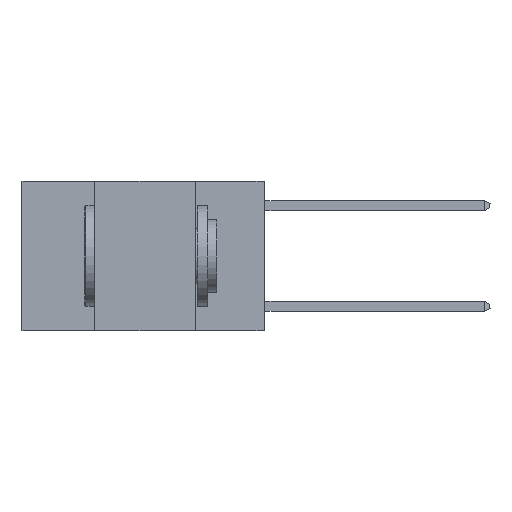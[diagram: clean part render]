
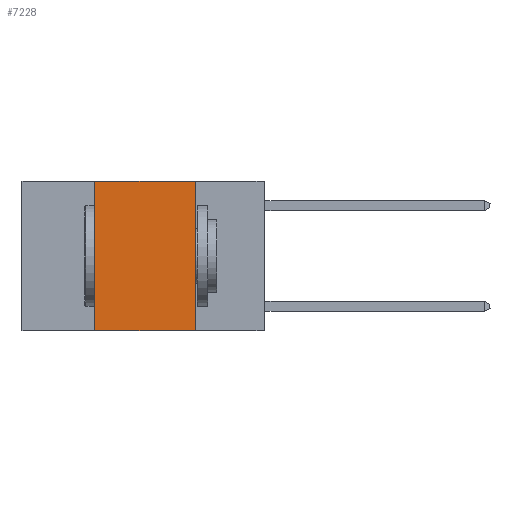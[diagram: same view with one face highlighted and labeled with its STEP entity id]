
A CAD part, left-side view. The second image highlights one B-rep face of the part: STEP entity #7228.
In plain terms, the highlighted planar face has unit normal (-1, 0, 0).
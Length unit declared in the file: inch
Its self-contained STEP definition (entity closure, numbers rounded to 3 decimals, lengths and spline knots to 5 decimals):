
#251 = VECTOR ( 'NONE', #2437, 39.37008 ) ;
#270 = EDGE_CURVE ( 'NONE', #9111, #2203, #6574, .T. ) ;
#506 = EDGE_LOOP ( 'NONE', ( #3416, #1735, #6594, #8773 ) ) ;
#583 = VECTOR ( 'NONE', #8448, 39.37008 ) ;
#635 = FACE_OUTER_BOUND ( 'NONE', #506, .T. ) ;
#727 = CARTESIAN_POINT ( 'NONE',  ( 0., 0.17, 0. ) ) ;
#1605 = CARTESIAN_POINT ( 'NONE',  ( 0., 0.17, -0.37 ) ) ;
#1732 = CARTESIAN_POINT ( 'NONE',  ( 0., 0.42, -0.37 ) ) ;
#1735 = ORIENTED_EDGE ( 'NONE', *, *, #2881, .F. ) ;
#2203 = VERTEX_POINT ( 'NONE', #5775 ) ;
#2244 = DIRECTION ( 'NONE',  ( 0., 0., 1. ) ) ;
#2437 = DIRECTION ( 'NONE',  ( 0., 0., -1. ) ) ;
#2881 = EDGE_CURVE ( 'NONE', #2203, #7790, #3238, .T. ) ;
#3238 = LINE ( 'NONE', #8332, #583 ) ;
#3416 = ORIENTED_EDGE ( 'NONE', *, *, #10229, .F. ) ;
#3858 = DIRECTION ( 'NONE',  ( 0., -1., 0. ) ) ;
#3930 = DIRECTION ( 'NONE',  ( 1., 0., 0. ) ) ;
#3982 = VECTOR ( 'NONE', #2244, 39.37008 ) ;
#4307 = VECTOR ( 'NONE', #3858, 39.37008 ) ;
#4714 = DIRECTION ( 'NONE',  ( 0., 0., -1. ) ) ;
#4939 = PLANE ( 'NONE',  #5691 ) ;
#5344 = LINE ( 'NONE', #9527, #251 ) ;
#5599 = CARTESIAN_POINT ( 'NONE',  ( 0., 0.6, -0.37 ) ) ;
#5691 = AXIS2_PLACEMENT_3D ( 'NONE', #7385, #3930, #4714 ) ;
#5775 = CARTESIAN_POINT ( 'NONE',  ( 0., 0.42, 0. ) ) ;
#6574 = LINE ( 'NONE', #10867, #3982 ) ;
#6594 = ORIENTED_EDGE ( 'NONE', *, *, #270, .F. ) ;
#7228 = ADVANCED_FACE ( 'NONE', ( #635 ), #4939, .F. ) ;
#7385 = CARTESIAN_POINT ( 'NONE',  ( 0., 0.6, 0. ) ) ;
#7790 = VERTEX_POINT ( 'NONE', #727 ) ;
#8332 = CARTESIAN_POINT ( 'NONE',  ( 0., 0.6, 0. ) ) ;
#8448 = DIRECTION ( 'NONE',  ( 0., -1., 0. ) ) ;
#8773 = ORIENTED_EDGE ( 'NONE', *, *, #10844, .T. ) ;
#8787 = LINE ( 'NONE', #5599, #4307 ) ;
#9111 = VERTEX_POINT ( 'NONE', #1732 ) ;
#9527 = CARTESIAN_POINT ( 'NONE',  ( 0., 0.17, 0. ) ) ;
#9935 = VERTEX_POINT ( 'NONE', #1605 ) ;
#10229 = EDGE_CURVE ( 'NONE', #7790, #9935, #5344, .T. ) ;
#10844 = EDGE_CURVE ( 'NONE', #9111, #9935, #8787, .T. ) ;
#10867 = CARTESIAN_POINT ( 'NONE',  ( 0., 0.42, 0. ) ) ;
